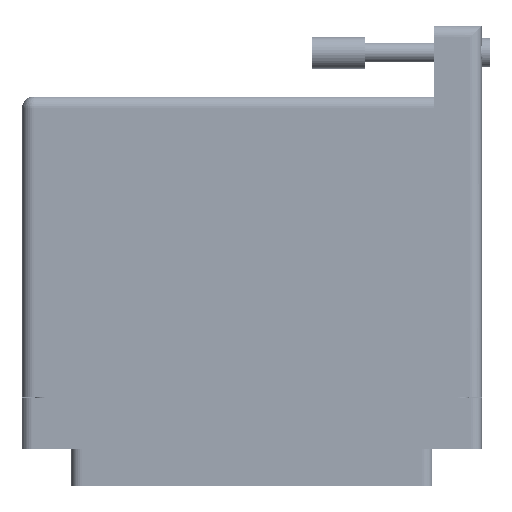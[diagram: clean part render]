
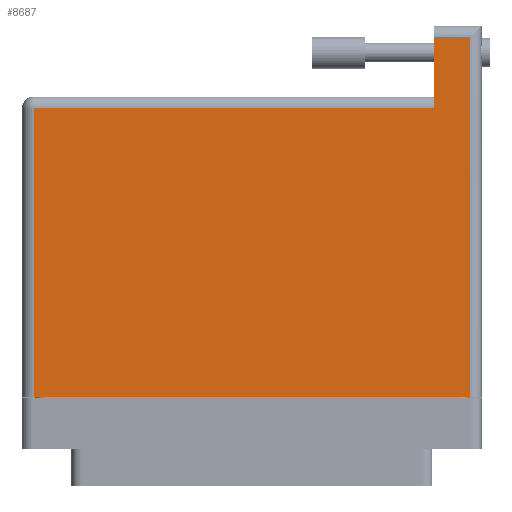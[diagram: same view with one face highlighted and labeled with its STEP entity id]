
A CAD part, front view. The second image highlights one B-rep face of the part: STEP entity #8687.
In plain terms, the highlighted face is planar.
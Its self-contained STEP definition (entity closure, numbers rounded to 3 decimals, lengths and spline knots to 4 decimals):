
#15 = ORIENTED_EDGE ( 'NONE', *, *, #7540, .T. ) ;
#1742 = LINE ( 'NONE', #35995, #35646 ) ;
#1980 = ORIENTED_EDGE ( 'NONE', *, *, #43986, .T. ) ;
#2236 = CARTESIAN_POINT ( 'NONE',  ( 1.079, 1.605, 0.617 ) ) ;
#4103 = CARTESIAN_POINT ( 'NONE',  ( -1.289, -0.1, 0.617 ) ) ;
#7540 = EDGE_CURVE ( 'NONE', #45348, #38910, #1742, .T. ) ;
#8154 = CARTESIAN_POINT ( 'NONE',  ( -1.359, -0.1, 0.617 ) ) ;
#8687 = ADVANCED_FACE ( 'NONE', ( #33386 ), #65235, .F. ) ;
#11612 = VECTOR ( 'NONE', #65853, 39.3701 ) ;
#12124 = ORIENTED_EDGE ( 'NONE', *, *, #58776, .T. ) ;
#12282 = ORIENTED_EDGE ( 'NONE', *, *, #70133, .T. ) ;
#12370 = EDGE_CURVE ( 'NONE', #59624, #41776, #28131, .T. ) ;
#15505 = CARTESIAN_POINT ( 'NONE',  ( -1.289, -0.1, 0.617 ) ) ;
#16571 = ORIENTED_EDGE ( 'NONE', *, *, #12370, .T. ) ;
#19241 = VECTOR ( 'NONE', #52895, 39.3701 ) ;
#24268 = DIRECTION ( 'NONE',  ( 1., 0., 0. ) ) ;
#25125 = DIRECTION ( 'NONE',  ( 0., 1., 0. ) ) ;
#25634 = CARTESIAN_POINT ( 'NONE',  ( 1.079, 2.095, 0.617 ) ) ;
#27677 = CARTESIAN_POINT ( 'NONE',  ( -1.359, 2.025, 0.617 ) ) ;
#28131 = LINE ( 'NONE', #68524, #34052 ) ;
#29514 = AXIS2_PLACEMENT_3D ( 'NONE', #48438, #54409, #37005 ) ;
#30279 = LINE ( 'NONE', #27677, #11612 ) ;
#31676 = VERTEX_POINT ( 'NONE', #53796 ) ;
#33386 = FACE_OUTER_BOUND ( 'NONE', #50465, .T. ) ;
#34052 = VECTOR ( 'NONE', #25125, 39.3701 ) ;
#34469 = LINE ( 'NONE', #25634, #19241 ) ;
#35646 = VECTOR ( 'NONE', #46067, 39.3701 ) ;
#35995 = CARTESIAN_POINT ( 'NONE',  ( -1.359, 1.605, 0.617 ) ) ;
#37005 = DIRECTION ( 'NONE',  ( -1., 0., 0. ) ) ;
#38910 = VERTEX_POINT ( 'NONE', #64071 ) ;
#41776 = VERTEX_POINT ( 'NONE', #58648 ) ;
#42019 = DIRECTION ( 'NONE',  ( 0., -1., 0. ) ) ;
#43986 = EDGE_CURVE ( 'NONE', #31676, #45348, #34469, .T. ) ;
#45348 = VERTEX_POINT ( 'NONE', #2236 ) ;
#46067 = DIRECTION ( 'NONE',  ( -1., 0., 0. ) ) ;
#48438 = CARTESIAN_POINT ( 'NONE',  ( -1.359, 1.675, 0.617 ) ) ;
#49613 = VECTOR ( 'NONE', #24268, 39.3701 ) ;
#50465 = EDGE_LOOP ( 'NONE', ( #15, #12124, #57440, #16571, #12282, #1980 ) ) ;
#52895 = DIRECTION ( 'NONE',  ( 0., -1., 0. ) ) ;
#53796 = CARTESIAN_POINT ( 'NONE',  ( 1.079, 2.025, 0.617 ) ) ;
#54409 = DIRECTION ( 'NONE',  ( 0., 0., -1. ) ) ;
#57440 = ORIENTED_EDGE ( 'NONE', *, *, #60752, .T. ) ;
#57612 = VERTEX_POINT ( 'NONE', #15505 ) ;
#57938 = CARTESIAN_POINT ( 'NONE',  ( 1.289, -0.1, 0.617 ) ) ;
#58648 = CARTESIAN_POINT ( 'NONE',  ( 1.289, 2.025, 0.617 ) ) ;
#58776 = EDGE_CURVE ( 'NONE', #38910, #57612, #69455, .T. ) ;
#59624 = VERTEX_POINT ( 'NONE', #57938 ) ;
#60752 = EDGE_CURVE ( 'NONE', #57612, #59624, #64041, .T. ) ;
#60922 = VECTOR ( 'NONE', #42019, 39.3701 ) ;
#64041 = LINE ( 'NONE', #8154, #49613 ) ;
#64071 = CARTESIAN_POINT ( 'NONE',  ( -1.289, 1.605, 0.617 ) ) ;
#65235 = PLANE ( 'NONE',  #29514 ) ;
#65853 = DIRECTION ( 'NONE',  ( -1., 0., 0. ) ) ;
#68524 = CARTESIAN_POINT ( 'NONE',  ( 1.289, 2.095, 0.617 ) ) ;
#69455 = LINE ( 'NONE', #4103, #60922 ) ;
#70133 = EDGE_CURVE ( 'NONE', #41776, #31676, #30279, .T. ) ;
